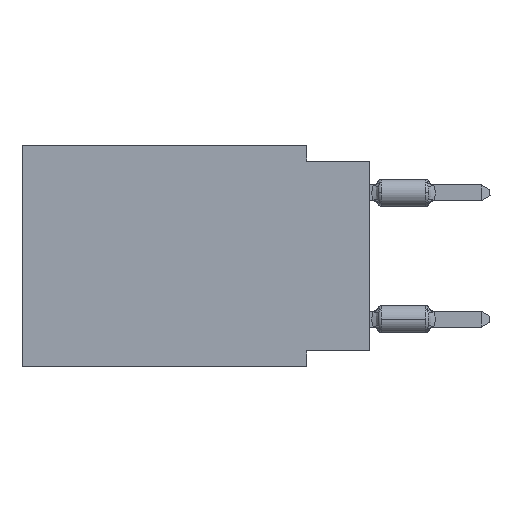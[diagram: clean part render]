
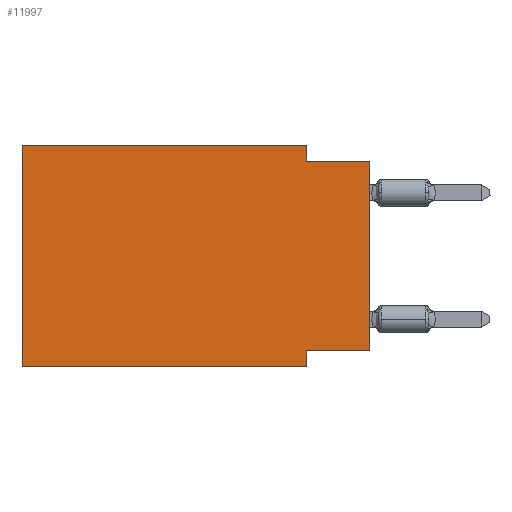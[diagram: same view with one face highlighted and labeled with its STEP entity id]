
A CAD part, left-side view. The second image highlights one B-rep face of the part: STEP entity #11997.
In plain terms, the highlighted planar face has unit normal (-1, 0, 0).
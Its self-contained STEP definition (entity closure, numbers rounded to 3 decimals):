
#462 = ORIENTED_EDGE ( 'NONE', *, *, #26053, .F. ) ;
#1258 = LINE ( 'NONE', #7767, #38651 ) ;
#1400 = DIRECTION ( 'NONE',  ( 0., -1., 0. ) ) ;
#1912 = DIRECTION ( 'NONE',  ( 0., 0., -1. ) ) ;
#2112 = CARTESIAN_POINT ( 'NONE',  ( 0., 13.97, -8.89 ) ) ;
#2228 = ORIENTED_EDGE ( 'NONE', *, *, #31829, .F. ) ;
#2959 = CARTESIAN_POINT ( 'NONE',  ( 0., 0., -8.255 ) ) ;
#3014 = ORIENTED_EDGE ( 'NONE', *, *, #21651, .F. ) ;
#4067 = VECTOR ( 'NONE', #45921, 1000. ) ;
#4241 = ORIENTED_EDGE ( 'NONE', *, *, #22717, .F. ) ;
#4800 = EDGE_CURVE ( 'NONE', #18706, #45628, #5003, .T. ) ;
#5003 = LINE ( 'NONE', #39639, #39335 ) ;
#6902 = DIRECTION ( 'NONE',  ( 0., 1., 0. ) ) ;
#7278 = VERTEX_POINT ( 'NONE', #24062 ) ;
#7767 = CARTESIAN_POINT ( 'NONE',  ( 0., 13.97, 0. ) ) ;
#9441 = VERTEX_POINT ( 'NONE', #43734 ) ;
#11997 = ADVANCED_FACE ( 'NONE', ( #37221 ), #26324, .F. ) ;
#12429 = EDGE_CURVE ( 'NONE', #9441, #26371, #37166, .T. ) ;
#13956 = CARTESIAN_POINT ( 'NONE',  ( 0., 2.54, 0. ) ) ;
#14037 = CARTESIAN_POINT ( 'NONE',  ( 0., 2.54, -8.89 ) ) ;
#18080 = VECTOR ( 'NONE', #44403, 1000. ) ;
#18706 = VERTEX_POINT ( 'NONE', #36690 ) ;
#19310 = EDGE_LOOP ( 'NONE', ( #19528, #3014, #2228, #32205, #462, #37861, #4241, #39623 ) ) ;
#19528 = ORIENTED_EDGE ( 'NONE', *, *, #4800, .T. ) ;
#19828 = LINE ( 'NONE', #27250, #37409 ) ;
#21476 = LINE ( 'NONE', #14037, #31551 ) ;
#21651 = EDGE_CURVE ( 'NONE', #39559, #45628, #19828, .T. ) ;
#22717 = EDGE_CURVE ( 'NONE', #44544, #7278, #21476, .T. ) ;
#22842 = DIRECTION ( 'NONE',  ( 1., 0., 0. ) ) ;
#24062 = CARTESIAN_POINT ( 'NONE',  ( 0., 2.54, -8.89 ) ) ;
#26053 = EDGE_CURVE ( 'NONE', #34095, #9441, #1258, .T. ) ;
#26324 = PLANE ( 'NONE',  #30787 ) ;
#26371 = VERTEX_POINT ( 'NONE', #13956 ) ;
#27073 = VECTOR ( 'NONE', #1400, 1000. ) ;
#27250 = CARTESIAN_POINT ( 'NONE',  ( 0., 0., -0.635 ) ) ;
#28942 = DIRECTION ( 'NONE',  ( 0., 0., 1. ) ) ;
#29555 = CARTESIAN_POINT ( 'NONE',  ( 0., 13.97, -8.89 ) ) ;
#30787 = AXIS2_PLACEMENT_3D ( 'NONE', #33745, #22842, #1912 ) ;
#31145 = LINE ( 'NONE', #2112, #18080 ) ;
#31307 = CARTESIAN_POINT ( 'NONE',  ( 0., 2.54, -8.255 ) ) ;
#31551 = VECTOR ( 'NONE', #45637, 1000. ) ;
#31829 = EDGE_CURVE ( 'NONE', #26371, #39559, #45244, .T. ) ;
#32205 = ORIENTED_EDGE ( 'NONE', *, *, #12429, .F. ) ;
#33026 = CARTESIAN_POINT ( 'NONE',  ( 0., 0., -0.635 ) ) ;
#33745 = CARTESIAN_POINT ( 'NONE',  ( 0., 13.97, 0. ) ) ;
#34095 = VERTEX_POINT ( 'NONE', #29555 ) ;
#34198 = DIRECTION ( 'NONE',  ( 0., -1., 0. ) ) ;
#34968 = CARTESIAN_POINT ( 'NONE',  ( 0., 2.54, -0.635 ) ) ;
#35474 = CARTESIAN_POINT ( 'NONE',  ( 0., 2.54, 0. ) ) ;
#36690 = CARTESIAN_POINT ( 'NONE',  ( 0., 0., -8.255 ) ) ;
#36775 = EDGE_CURVE ( 'NONE', #34095, #7278, #31145, .T. ) ;
#37166 = LINE ( 'NONE', #40448, #27073 ) ;
#37221 = FACE_OUTER_BOUND ( 'NONE', #19310, .T. ) ;
#37332 = EDGE_CURVE ( 'NONE', #18706, #44544, #42024, .T. ) ;
#37409 = VECTOR ( 'NONE', #34198, 1000. ) ;
#37861 = ORIENTED_EDGE ( 'NONE', *, *, #36775, .T. ) ;
#38302 = VECTOR ( 'NONE', #6902, 1000. ) ;
#38651 = VECTOR ( 'NONE', #43767, 1000. ) ;
#39335 = VECTOR ( 'NONE', #28942, 1000. ) ;
#39559 = VERTEX_POINT ( 'NONE', #34968 ) ;
#39623 = ORIENTED_EDGE ( 'NONE', *, *, #37332, .F. ) ;
#39639 = CARTESIAN_POINT ( 'NONE',  ( 0., 0., 0. ) ) ;
#40448 = CARTESIAN_POINT ( 'NONE',  ( 0., 13.97, 0. ) ) ;
#42024 = LINE ( 'NONE', #2959, #38302 ) ;
#43734 = CARTESIAN_POINT ( 'NONE',  ( 0., 13.97, 0. ) ) ;
#43767 = DIRECTION ( 'NONE',  ( 0., 0., 1. ) ) ;
#44403 = DIRECTION ( 'NONE',  ( 0., -1., 0. ) ) ;
#44544 = VERTEX_POINT ( 'NONE', #31307 ) ;
#45244 = LINE ( 'NONE', #35474, #4067 ) ;
#45628 = VERTEX_POINT ( 'NONE', #33026 ) ;
#45637 = DIRECTION ( 'NONE',  ( 0., 0., -1. ) ) ;
#45921 = DIRECTION ( 'NONE',  ( 0., 0., -1. ) ) ;
